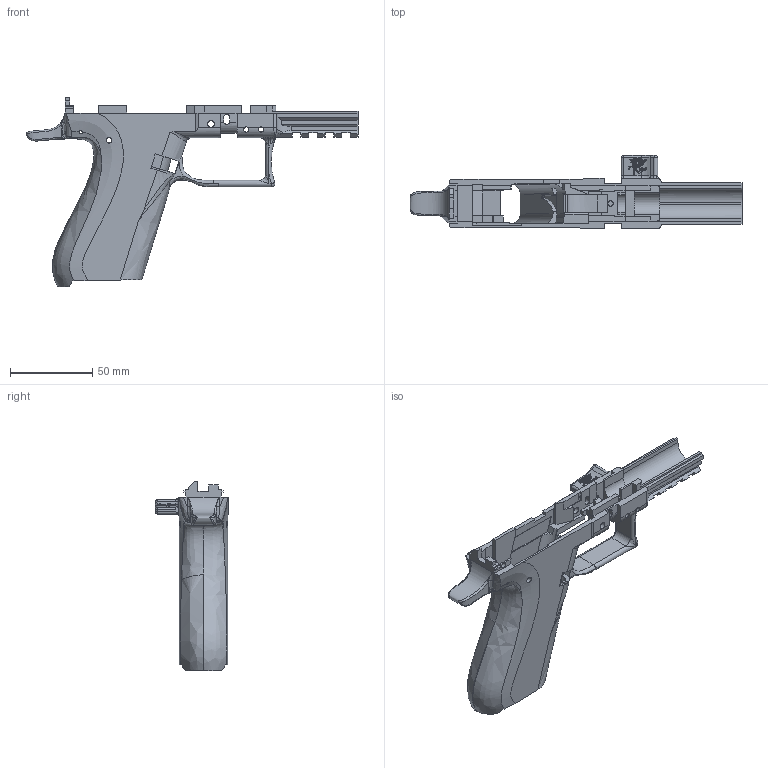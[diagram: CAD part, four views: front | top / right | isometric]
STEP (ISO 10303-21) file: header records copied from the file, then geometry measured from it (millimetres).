
FILE_DESCRIPTION(/* description */ (''),/* implementation_level */ '2;1');
FILE_NAME(/* name */ 'P99 Frame 1204 Match v3.step',/* time_stamp */ '2022-05-06T11:44:25-04:00',/* author */ (''),/* organization */ (''),/* preprocessor_version */ 'ST-DEVELOPER v18.1',/* originating_system */ 'Autodesk Translation Framework v10.14.0.1471',/* authorisation */ '');
FILE_SCHEMA (('AUTOMOTIVE_DESIGN { 1 0 10303 214 3 1 1 }'));
Length unit declared in the file: millimetre
Products named in the file (1): P99 Frame 1204 Match
Bounding box: 202.19 x 44.5 x 115.7 mm (x, y, z)
Volume: 88238.8 mm3; surface area: 49659.4 mm2
Topology: 1 solids, 1 shells, 1446 faces, 4223 edges, 2786 vertices
Faces by surface type: bspline 930, plane 419, cylinder 83, torus 8, sphere 6
Full cylindrical faces by diameter (mm): 0.8 x1, 1.7 x1, 2 x2, 3.2 x5, 3.3 x1, 3.4 x2, 4.1 x2
Entity records: 71123 total; most frequent: CARTESIAN_POINT 40872, ORIENTED_EDGE 8426, EDGE_CURVE 4213, DIRECTION 3576, VERTEX_POINT 2786, LINE 1980, VECTOR 1980, EDGE_LOOP 1501
